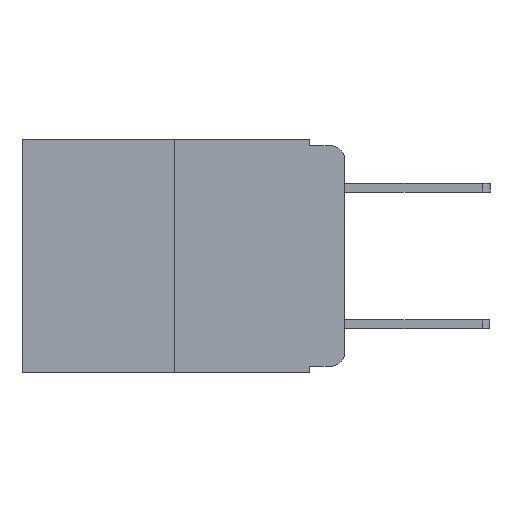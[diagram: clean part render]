
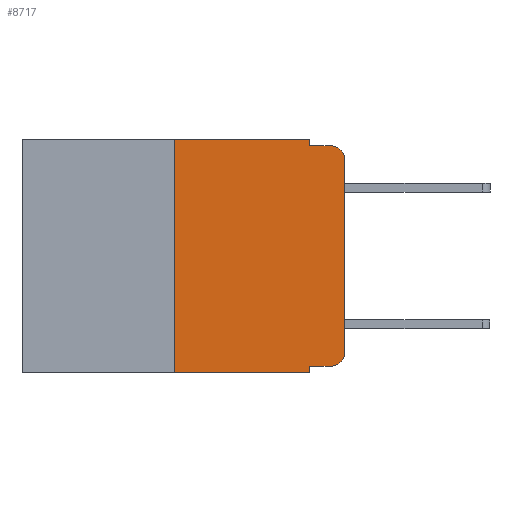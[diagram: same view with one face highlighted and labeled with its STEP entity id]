
A CAD part, left-side view. The second image highlights one B-rep face of the part: STEP entity #8717.
In plain terms, the highlighted planar face has unit normal (-1, 0, 0).
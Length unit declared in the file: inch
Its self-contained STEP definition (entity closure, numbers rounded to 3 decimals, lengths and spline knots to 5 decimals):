
#51 = VERTEX_POINT ( 'NONE', #7844 ) ;
#252 = CARTESIAN_POINT ( 'NONE',  ( 0., 0.473, 0. ) ) ;
#434 = DIRECTION ( 'NONE',  ( 0., 0., -1. ) ) ;
#510 = ORIENTED_EDGE ( 'NONE', *, *, #9473, .F. ) ;
#570 = CARTESIAN_POINT ( 'NONE',  ( 0., 0.051, -0.333 ) ) ;
#576 = CARTESIAN_POINT ( 'NONE',  ( 0., 0.473, 0. ) ) ;
#706 = EDGE_LOOP ( 'NONE', ( #967, #9207, #4493, #510, #3714, #8772, #6587, #4342, #4652, #4965 ) ) ;
#967 = ORIENTED_EDGE ( 'NONE', *, *, #2216, .T. ) ;
#1232 = DIRECTION ( 'NONE',  ( 0., 0., -1. ) ) ;
#1261 = AXIS2_PLACEMENT_3D ( 'NONE', #8429, #2709, #9357 ) ;
#1375 = CARTESIAN_POINT ( 'NONE',  ( 0., 0., 0. ) ) ;
#1631 = LINE ( 'NONE', #11666, #11389 ) ;
#1688 = EDGE_CURVE ( 'NONE', #6608, #4195, #6708, .T. ) ;
#1810 = EDGE_CURVE ( 'NONE', #3458, #11044, #5285, .T. ) ;
#2216 = EDGE_CURVE ( 'NONE', #11044, #51, #7780, .T. ) ;
#2451 = LINE ( 'NONE', #11273, #4754 ) ;
#2709 = DIRECTION ( 'NONE',  ( -1., 0., 0. ) ) ;
#2762 = CIRCLE ( 'NONE', #7488, 0.02 ) ;
#2839 = VERTEX_POINT ( 'NONE', #10657 ) ;
#2866 = VERTEX_POINT ( 'NONE', #6072 ) ;
#3116 = EDGE_CURVE ( 'NONE', #5824, #3458, #6855, .T. ) ;
#3167 = PLANE ( 'NONE',  #5802 ) ;
#3256 = LINE ( 'NONE', #3392, #10484 ) ;
#3261 = DIRECTION ( 'NONE',  ( 0., 0., 1. ) ) ;
#3324 = CARTESIAN_POINT ( 'NONE',  ( 0., 0.02, -0.333 ) ) ;
#3326 = CARTESIAN_POINT ( 'NONE',  ( 0., 0., -0.313 ) ) ;
#3380 = CARTESIAN_POINT ( 'NONE',  ( 0., 0.051, 0. ) ) ;
#3392 = CARTESIAN_POINT ( 'NONE',  ( 0., 0.051, 0. ) ) ;
#3458 = VERTEX_POINT ( 'NONE', #3324 ) ;
#3697 = VERTEX_POINT ( 'NONE', #6552 ) ;
#3714 = ORIENTED_EDGE ( 'NONE', *, *, #1688, .F. ) ;
#4041 = FACE_OUTER_BOUND ( 'NONE', #706, .T. ) ;
#4195 = VERTEX_POINT ( 'NONE', #3380 ) ;
#4342 = ORIENTED_EDGE ( 'NONE', *, *, #6347, .F. ) ;
#4493 = ORIENTED_EDGE ( 'NONE', *, *, #10087, .F. ) ;
#4652 = ORIENTED_EDGE ( 'NONE', *, *, #3116, .T. ) ;
#4754 = VECTOR ( 'NONE', #12154, 39.37008 ) ;
#4774 = DIRECTION ( 'NONE',  ( 0., -1., 0. ) ) ;
#4965 = ORIENTED_EDGE ( 'NONE', *, *, #1810, .T. ) ;
#5274 = VECTOR ( 'NONE', #7146, 39.37008 ) ;
#5285 = CIRCLE ( 'NONE', #1261, 0.02 ) ;
#5309 = DIRECTION ( 'NONE',  ( 0., -1., 0. ) ) ;
#5663 = VECTOR ( 'NONE', #5309, 39.37008 ) ;
#5681 = CARTESIAN_POINT ( 'NONE',  ( 0., 0.02, -0.03 ) ) ;
#5802 = AXIS2_PLACEMENT_3D ( 'NONE', #252, #7018, #1232 ) ;
#5824 = VERTEX_POINT ( 'NONE', #570 ) ;
#5918 = LINE ( 'NONE', #11758, #10564 ) ;
#6072 = CARTESIAN_POINT ( 'NONE',  ( 0., 0.051, -0.343 ) ) ;
#6347 = EDGE_CURVE ( 'NONE', #5824, #2866, #5918, .T. ) ;
#6410 = VECTOR ( 'NONE', #11889, 39.37008 ) ;
#6552 = CARTESIAN_POINT ( 'NONE',  ( 0., 0.25, -0.343 ) ) ;
#6587 = ORIENTED_EDGE ( 'NONE', *, *, #11356, .T. ) ;
#6608 = VERTEX_POINT ( 'NONE', #8446 ) ;
#6642 = DIRECTION ( 'NONE',  ( 0., 0., -1. ) ) ;
#6708 = LINE ( 'NONE', #576, #6410 ) ;
#6855 = LINE ( 'NONE', #9446, #10898 ) ;
#7018 = DIRECTION ( 'NONE',  ( 1., 0., 0. ) ) ;
#7146 = DIRECTION ( 'NONE',  ( 0., 0., 1. ) ) ;
#7488 = AXIS2_PLACEMENT_3D ( 'NONE', #5681, #12121, #6642 ) ;
#7616 = EDGE_CURVE ( 'NONE', #3697, #6608, #1631, .T. ) ;
#7780 = LINE ( 'NONE', #1375, #5274 ) ;
#7844 = CARTESIAN_POINT ( 'NONE',  ( 0., 0., -0.03 ) ) ;
#8137 = CARTESIAN_POINT ( 'NONE',  ( 0., 0.051, -0.01 ) ) ;
#8429 = CARTESIAN_POINT ( 'NONE',  ( 0., 0.02, -0.313 ) ) ;
#8446 = CARTESIAN_POINT ( 'NONE',  ( 0., 0.25, 0. ) ) ;
#8717 = ADVANCED_FACE ( 'NONE', ( #4041 ), #3167, .F. ) ;
#8772 = ORIENTED_EDGE ( 'NONE', *, *, #7616, .F. ) ;
#9080 = DIRECTION ( 'NONE',  ( 0., 0., -1. ) ) ;
#9207 = ORIENTED_EDGE ( 'NONE', *, *, #11302, .T. ) ;
#9357 = DIRECTION ( 'NONE',  ( 0., 0., -1. ) ) ;
#9446 = CARTESIAN_POINT ( 'NONE',  ( 0., 0.051, -0.333 ) ) ;
#9473 = EDGE_CURVE ( 'NONE', #4195, #2839, #3256, .T. ) ;
#10087 = EDGE_CURVE ( 'NONE', #2839, #10747, #10599, .T. ) ;
#10484 = VECTOR ( 'NONE', #9080, 39.37008 ) ;
#10564 = VECTOR ( 'NONE', #434, 39.37008 ) ;
#10599 = LINE ( 'NONE', #8137, #5663 ) ;
#10657 = CARTESIAN_POINT ( 'NONE',  ( 0., 0.051, -0.01 ) ) ;
#10747 = VERTEX_POINT ( 'NONE', #11823 ) ;
#10898 = VECTOR ( 'NONE', #4774, 39.37008 ) ;
#11044 = VERTEX_POINT ( 'NONE', #3326 ) ;
#11273 = CARTESIAN_POINT ( 'NONE',  ( 0., 0.473, -0.343 ) ) ;
#11302 = EDGE_CURVE ( 'NONE', #51, #10747, #2762, .T. ) ;
#11356 = EDGE_CURVE ( 'NONE', #3697, #2866, #2451, .T. ) ;
#11389 = VECTOR ( 'NONE', #3261, 39.37008 ) ;
#11666 = CARTESIAN_POINT ( 'NONE',  ( 0., 0.25, 0. ) ) ;
#11758 = CARTESIAN_POINT ( 'NONE',  ( 0., 0.051, 0. ) ) ;
#11823 = CARTESIAN_POINT ( 'NONE',  ( 0., 0.02, -0.01 ) ) ;
#11889 = DIRECTION ( 'NONE',  ( 0., -1., 0. ) ) ;
#12121 = DIRECTION ( 'NONE',  ( -1., 0., 0. ) ) ;
#12154 = DIRECTION ( 'NONE',  ( 0., -1., 0. ) ) ;
